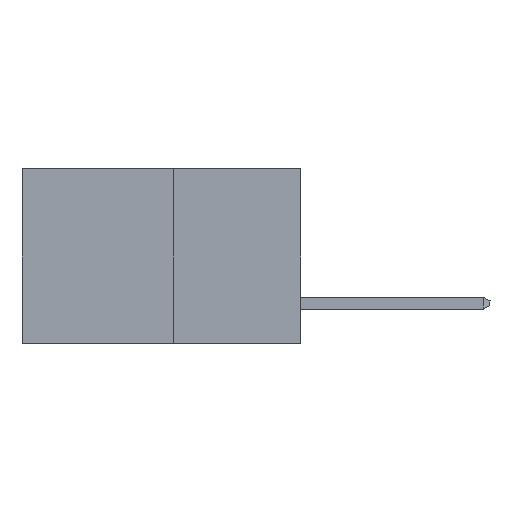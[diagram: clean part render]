
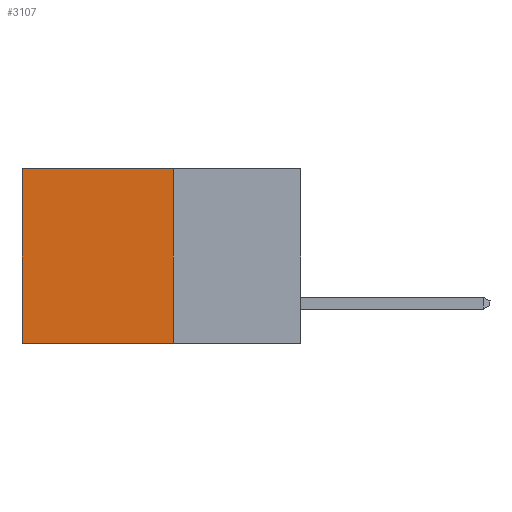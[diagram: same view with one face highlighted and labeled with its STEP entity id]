
A CAD part, left-side view. The second image highlights one B-rep face of the part: STEP entity #3107.
In plain terms, the highlighted planar face has unit normal (-1, 0, 0).
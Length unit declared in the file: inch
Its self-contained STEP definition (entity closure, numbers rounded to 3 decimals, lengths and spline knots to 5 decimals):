
#148 = LINE ( 'NONE', #8051, #4633 ) ;
#278 = FACE_OUTER_BOUND ( 'NONE', #5946, .T. ) ;
#599 = AXIS2_PLACEMENT_3D ( 'NONE', #5652, #10608, #10568 ) ;
#629 = DIRECTION ( 'NONE',  ( 0., 0., -1. ) ) ;
#631 = CARTESIAN_POINT ( 'NONE',  ( 0.277, 0.59, -0.37 ) ) ;
#652 = DIRECTION ( 'NONE',  ( 0., 0., -1. ) ) ;
#715 = EDGE_CURVE ( 'NONE', #1571, #6863, #3747, .T. ) ;
#1571 = VERTEX_POINT ( 'NONE', #8247 ) ;
#1652 = CARTESIAN_POINT ( 'NONE',  ( 0.277, 0.27, 0. ) ) ;
#1804 = DIRECTION ( 'NONE',  ( 0., 1., 0. ) ) ;
#2458 = EDGE_CURVE ( 'NONE', #8921, #1571, #148, .T. ) ;
#2650 = DIRECTION ( 'NONE',  ( 0., 1., 0. ) ) ;
#2685 = CARTESIAN_POINT ( 'NONE',  ( 0.277, 0.27, 0. ) ) ;
#3107 = ADVANCED_FACE ( 'NONE', ( #278 ), #4043, .F. ) ;
#3475 = VECTOR ( 'NONE', #1804, 39.37008 ) ;
#3747 = LINE ( 'NONE', #4776, #3475 ) ;
#3748 = VERTEX_POINT ( 'NONE', #10698 ) ;
#4043 = PLANE ( 'NONE',  #599 ) ;
#4143 = EDGE_CURVE ( 'NONE', #3748, #6863, #6325, .T. ) ;
#4633 = VECTOR ( 'NONE', #652, 39.37008 ) ;
#4776 = CARTESIAN_POINT ( 'NONE',  ( 0.277, 0.27, -0.37 ) ) ;
#4849 = CARTESIAN_POINT ( 'NONE',  ( 0.277, 0.59, -0.37 ) ) ;
#5652 = CARTESIAN_POINT ( 'NONE',  ( 0.277, 0.27, -0.37 ) ) ;
#5946 = EDGE_LOOP ( 'NONE', ( #8603, #10141, #10134, #10122 ) ) ;
#6325 = LINE ( 'NONE', #631, #10306 ) ;
#6863 = VERTEX_POINT ( 'NONE', #4849 ) ;
#7939 = EDGE_CURVE ( 'NONE', #8921, #3748, #10362, .T. ) ;
#8051 = CARTESIAN_POINT ( 'NONE',  ( 0.277, 0.27, -0.37 ) ) ;
#8194 = VECTOR ( 'NONE', #2650, 39.37008 ) ;
#8247 = CARTESIAN_POINT ( 'NONE',  ( 0.277, 0.27, -0.37 ) ) ;
#8603 = ORIENTED_EDGE ( 'NONE', *, *, #4143, .T. ) ;
#8921 = VERTEX_POINT ( 'NONE', #1652 ) ;
#10122 = ORIENTED_EDGE ( 'NONE', *, *, #7939, .T. ) ;
#10134 = ORIENTED_EDGE ( 'NONE', *, *, #2458, .F. ) ;
#10141 = ORIENTED_EDGE ( 'NONE', *, *, #715, .F. ) ;
#10306 = VECTOR ( 'NONE', #629, 39.37008 ) ;
#10362 = LINE ( 'NONE', #2685, #8194 ) ;
#10568 = DIRECTION ( 'NONE',  ( 0., 0., -1. ) ) ;
#10608 = DIRECTION ( 'NONE',  ( 1., 0., 0. ) ) ;
#10698 = CARTESIAN_POINT ( 'NONE',  ( 0.277, 0.59, 0. ) ) ;
